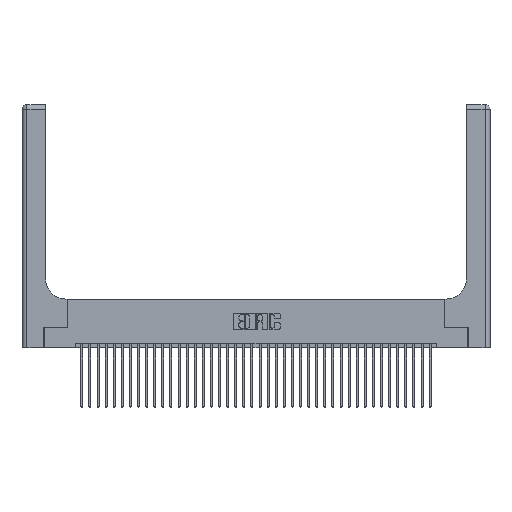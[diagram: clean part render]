
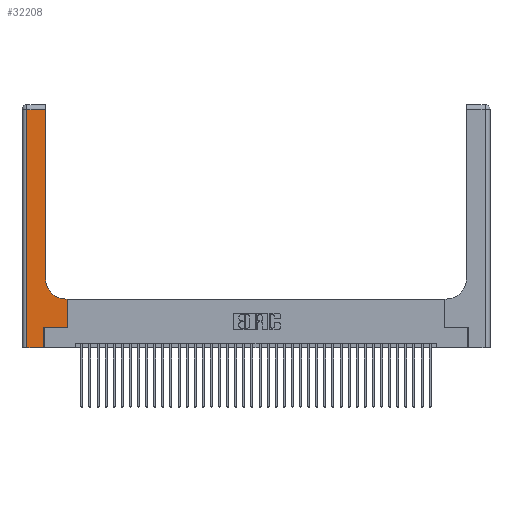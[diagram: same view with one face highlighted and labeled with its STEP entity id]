
A CAD part, top view. The second image highlights one B-rep face of the part: STEP entity #32208.
In plain terms, the highlighted planar face has unit normal (0, 0, 1).
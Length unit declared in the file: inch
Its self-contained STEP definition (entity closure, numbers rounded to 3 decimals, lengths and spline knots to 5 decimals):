
#2920 = VECTOR ( 'NONE', #26629, 39.37008 ) ;
#3843 = CIRCLE ( 'NONE', #29480, 0.25 ) ;
#4341 = EDGE_CURVE ( 'NONE', #32516, #29353, #9327, .T. ) ;
#5106 = PLANE ( 'NONE',  #18061 ) ;
#5118 = CARTESIAN_POINT ( 'NONE',  ( 0.269, 0.25, 0.37 ) ) ;
#6065 = DIRECTION ( 'NONE',  ( 1., 0., 0. ) ) ;
#6307 = DIRECTION ( 'NONE',  ( 0., 1., 0. ) ) ;
#6433 = LINE ( 'NONE', #24269, #21708 ) ;
#6529 = CARTESIAN_POINT ( 'NONE',  ( 0.5585, 0.6, 0.37 ) ) ;
#6615 = EDGE_LOOP ( 'NONE', ( #16381, #8421, #18501, #7064, #30934, #28898, #27841, #13030, #20958 ) ) ;
#6962 = VECTOR ( 'NONE', #6065, 39.37008 ) ;
#7064 = ORIENTED_EDGE ( 'NONE', *, *, #4341, .T. ) ;
#7272 = VERTEX_POINT ( 'NONE', #15516 ) ;
#7718 = VERTEX_POINT ( 'NONE', #27064 ) ;
#8421 = ORIENTED_EDGE ( 'NONE', *, *, #22766, .T. ) ;
#9327 = LINE ( 'NONE', #21285, #6962 ) ;
#10218 = VERTEX_POINT ( 'NONE', #5118 ) ;
#11637 = VECTOR ( 'NONE', #13521, 39.37008 ) ;
#12084 = DIRECTION ( 'NONE',  ( 0., 0., -1. ) ) ;
#12213 = CARTESIAN_POINT ( 'NONE',  ( 0.2915, 3., 0.37 ) ) ;
#12477 = LINE ( 'NONE', #34638, #21485 ) ;
#12566 = VERTEX_POINT ( 'NONE', #27365 ) ;
#12607 = VERTEX_POINT ( 'NONE', #21763 ) ;
#13030 = ORIENTED_EDGE ( 'NONE', *, *, #28850, .T. ) ;
#13031 = CARTESIAN_POINT ( 'NONE',  ( 0.269, 0., 0.37 ) ) ;
#13521 = DIRECTION ( 'NONE',  ( 0., 1., 0. ) ) ;
#14432 = VECTOR ( 'NONE', #17559, 39.37008 ) ;
#14987 = VECTOR ( 'NONE', #6307, 39.37008 ) ;
#15516 = CARTESIAN_POINT ( 'NONE',  ( 0.2915, 0.85, 0.37 ) ) ;
#16381 = ORIENTED_EDGE ( 'NONE', *, *, #20633, .T. ) ;
#17559 = DIRECTION ( 'NONE',  ( -1., 0., 0. ) ) ;
#17815 = DIRECTION ( 'NONE',  ( 1., 0., 0. ) ) ;
#18061 = AXIS2_PLACEMENT_3D ( 'NONE', #26952, #32402, #20430 ) ;
#18260 = LINE ( 'NONE', #20621, #14432 ) ;
#18501 = ORIENTED_EDGE ( 'NONE', *, *, #30931, .T. ) ;
#19281 = LINE ( 'NONE', #12213, #14987 ) ;
#20430 = DIRECTION ( 'NONE',  ( -1., 0., 0. ) ) ;
#20471 = VECTOR ( 'NONE', #39402, 39.37008 ) ;
#20621 = CARTESIAN_POINT ( 'NONE',  ( 0.2915, 0.6, 0.37 ) ) ;
#20633 = EDGE_CURVE ( 'NONE', #7272, #12566, #19281, .T. ) ;
#20958 = ORIENTED_EDGE ( 'NONE', *, *, #23440, .T. ) ;
#21285 = CARTESIAN_POINT ( 'NONE',  ( 0., 0., 0.37 ) ) ;
#21485 = VECTOR ( 'NONE', #31858, 39.37008 ) ;
#21708 = VECTOR ( 'NONE', #36022, 39.37008 ) ;
#21763 = CARTESIAN_POINT ( 'NONE',  ( 0.5585, 0.25, 0.37 ) ) ;
#22766 = EDGE_CURVE ( 'NONE', #12566, #7718, #25339, .T. ) ;
#23440 = EDGE_CURVE ( 'NONE', #36000, #7272, #3843, .T. ) ;
#23672 = CARTESIAN_POINT ( 'NONE',  ( 0.06, 3., 0.37 ) ) ;
#24269 = CARTESIAN_POINT ( 'NONE',  ( 0.5585, 0.25, 0.37 ) ) ;
#25339 = LINE ( 'NONE', #33278, #2920 ) ;
#26199 = EDGE_CURVE ( 'NONE', #10218, #12607, #12477, .T. ) ;
#26629 = DIRECTION ( 'NONE',  ( -1., 0., 0. ) ) ;
#26952 = CARTESIAN_POINT ( 'NONE',  ( 0., 3., 0.37 ) ) ;
#27064 = CARTESIAN_POINT ( 'NONE',  ( 0.06, 2.94, 0.37 ) ) ;
#27365 = CARTESIAN_POINT ( 'NONE',  ( 0.2915, 2.94, 0.37 ) ) ;
#27622 = EDGE_CURVE ( 'NONE', #29353, #10218, #28819, .T. ) ;
#27841 = ORIENTED_EDGE ( 'NONE', *, *, #36578, .T. ) ;
#28819 = LINE ( 'NONE', #31762, #11637 ) ;
#28850 = EDGE_CURVE ( 'NONE', #32492, #36000, #18260, .T. ) ;
#28898 = ORIENTED_EDGE ( 'NONE', *, *, #26199, .T. ) ;
#29353 = VERTEX_POINT ( 'NONE', #13031 ) ;
#29480 = AXIS2_PLACEMENT_3D ( 'NONE', #39263, #12084, #17815 ) ;
#30240 = CARTESIAN_POINT ( 'NONE',  ( 0.5415, 0.6, 0.37 ) ) ;
#30931 = EDGE_CURVE ( 'NONE', #7718, #32516, #38596, .T. ) ;
#30934 = ORIENTED_EDGE ( 'NONE', *, *, #27622, .T. ) ;
#31762 = CARTESIAN_POINT ( 'NONE',  ( 0.269, 0., 0.37 ) ) ;
#31858 = DIRECTION ( 'NONE',  ( 1., 0., 0. ) ) ;
#32208 = ADVANCED_FACE ( 'NONE', ( #32731 ), #5106, .F. ) ;
#32402 = DIRECTION ( 'NONE',  ( 0., 0., -1. ) ) ;
#32492 = VERTEX_POINT ( 'NONE', #6529 ) ;
#32516 = VERTEX_POINT ( 'NONE', #34894 ) ;
#32731 = FACE_OUTER_BOUND ( 'NONE', #6615, .T. ) ;
#33278 = CARTESIAN_POINT ( 'NONE',  ( 0., 2.94, 0.37 ) ) ;
#34638 = CARTESIAN_POINT ( 'NONE',  ( 0.269, 0.25, 0.37 ) ) ;
#34894 = CARTESIAN_POINT ( 'NONE',  ( 0.06, 0., 0.37 ) ) ;
#36000 = VERTEX_POINT ( 'NONE', #30240 ) ;
#36022 = DIRECTION ( 'NONE',  ( 0., 1., 0. ) ) ;
#36578 = EDGE_CURVE ( 'NONE', #12607, #32492, #6433, .T. ) ;
#38596 = LINE ( 'NONE', #23672, #20471 ) ;
#39263 = CARTESIAN_POINT ( 'NONE',  ( 0.5415, 0.85, 0.37 ) ) ;
#39402 = DIRECTION ( 'NONE',  ( 0., -1., 0. ) ) ;
